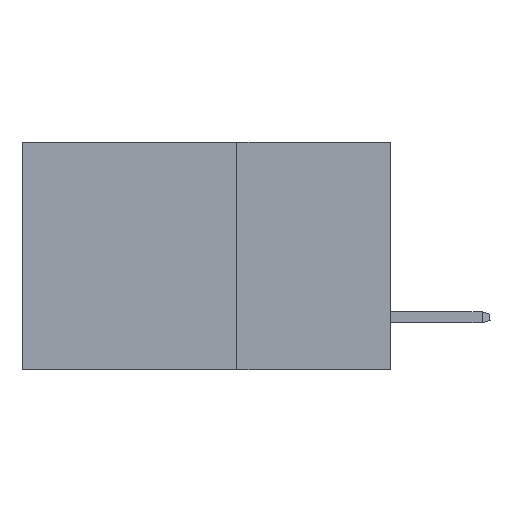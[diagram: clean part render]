
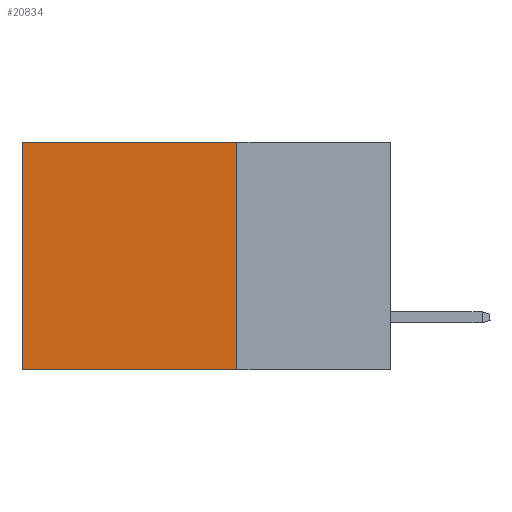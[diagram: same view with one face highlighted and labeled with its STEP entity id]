
A CAD part, left-side view. The second image highlights one B-rep face of the part: STEP entity #20834.
In plain terms, the highlighted planar face has unit normal (-1, 0, 0).
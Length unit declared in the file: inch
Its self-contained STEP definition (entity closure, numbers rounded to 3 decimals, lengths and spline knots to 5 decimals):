
#2408 = VERTEX_POINT ( 'NONE', #42140 ) ;
#2976 = CARTESIAN_POINT ( 'NONE',  ( 0.2875, 0.6, 0. ) ) ;
#3122 = DIRECTION ( 'NONE',  ( 0., 0., -1. ) ) ;
#3639 = CARTESIAN_POINT ( 'NONE',  ( 0.2875, 0.25, -0.37 ) ) ;
#4031 = DIRECTION ( 'NONE',  ( 0., 1., 0. ) ) ;
#4212 = VECTOR ( 'NONE', #43320, 39.37008 ) ;
#4613 = DIRECTION ( 'NONE',  ( 0., 0., -1. ) ) ;
#5276 = LINE ( 'NONE', #42897, #49406 ) ;
#8156 = AXIS2_PLACEMENT_3D ( 'NONE', #20809, #38853, #4613 ) ;
#8592 = LINE ( 'NONE', #17525, #28779 ) ;
#8737 = PLANE ( 'NONE',  #8156 ) ;
#10779 = LINE ( 'NONE', #42156, #37743 ) ;
#11421 = FACE_OUTER_BOUND ( 'NONE', #45479, .T. ) ;
#12560 = VERTEX_POINT ( 'NONE', #2976 ) ;
#13507 = VERTEX_POINT ( 'NONE', #16837 ) ;
#14211 = DIRECTION ( 'NONE',  ( 0., 0., -1. ) ) ;
#16193 = EDGE_CURVE ( 'NONE', #13507, #12560, #5276, .T. ) ;
#16747 = EDGE_CURVE ( 'NONE', #12560, #2408, #10779, .T. ) ;
#16837 = CARTESIAN_POINT ( 'NONE',  ( 0.2875, 0.25, 0. ) ) ;
#17525 = CARTESIAN_POINT ( 'NONE',  ( 0.2875, 0.25, 0. ) ) ;
#18031 = ORIENTED_EDGE ( 'NONE', *, *, #16747, .T. ) ;
#20809 = CARTESIAN_POINT ( 'NONE',  ( 0.2875, 0.25, 0. ) ) ;
#20834 = ADVANCED_FACE ( 'NONE', ( #11421 ), #8737, .F. ) ;
#23521 = CARTESIAN_POINT ( 'NONE',  ( 0.2875, 0.25, -0.37 ) ) ;
#26899 = VERTEX_POINT ( 'NONE', #3639 ) ;
#28240 = ORIENTED_EDGE ( 'NONE', *, *, #38169, .F. ) ;
#28779 = VECTOR ( 'NONE', #14211, 39.37008 ) ;
#32428 = LINE ( 'NONE', #23521, #4212 ) ;
#37743 = VECTOR ( 'NONE', #3122, 39.37008 ) ;
#38169 = EDGE_CURVE ( 'NONE', #26899, #2408, #32428, .T. ) ;
#38853 = DIRECTION ( 'NONE',  ( 1., 0., 0. ) ) ;
#42140 = CARTESIAN_POINT ( 'NONE',  ( 0.2875, 0.6, -0.37 ) ) ;
#42156 = CARTESIAN_POINT ( 'NONE',  ( 0.2875, 0.6, 0. ) ) ;
#42897 = CARTESIAN_POINT ( 'NONE',  ( 0.2875, 0.25, 0. ) ) ;
#43320 = DIRECTION ( 'NONE',  ( 0., 1., 0. ) ) ;
#43834 = ORIENTED_EDGE ( 'NONE', *, *, #46383, .F. ) ;
#45479 = EDGE_LOOP ( 'NONE', ( #18031, #28240, #43834, #50717 ) ) ;
#46383 = EDGE_CURVE ( 'NONE', #13507, #26899, #8592, .T. ) ;
#49406 = VECTOR ( 'NONE', #4031, 39.37008 ) ;
#50717 = ORIENTED_EDGE ( 'NONE', *, *, #16193, .T. ) ;
